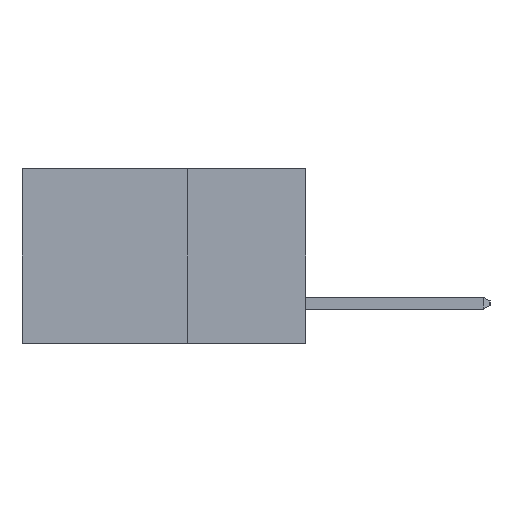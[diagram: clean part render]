
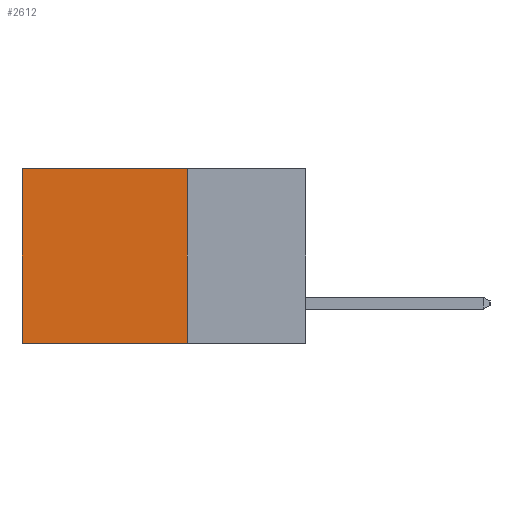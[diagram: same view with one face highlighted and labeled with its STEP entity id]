
A CAD part, left-side view. The second image highlights one B-rep face of the part: STEP entity #2612.
In plain terms, the highlighted planar face has unit normal (-1, 0, 0).
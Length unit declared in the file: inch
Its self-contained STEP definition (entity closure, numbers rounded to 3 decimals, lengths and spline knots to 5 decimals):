
#18 = CARTESIAN_POINT ( 'NONE',  ( 0.298, 0.25, 0. ) ) ;
#337 = DIRECTION ( 'NONE',  ( 0., 0., -1. ) ) ;
#370 = ORIENTED_EDGE ( 'NONE', *, *, #6235, .F. ) ;
#960 = DIRECTION ( 'NONE',  ( 0., 0., -1. ) ) ;
#2028 = VECTOR ( 'NONE', #3389, 39.37008 ) ;
#2294 = LINE ( 'NONE', #2478, #2028 ) ;
#2448 = FACE_OUTER_BOUND ( 'NONE', #9030, .T. ) ;
#2453 = PLANE ( 'NONE',  #4534 ) ;
#2478 = CARTESIAN_POINT ( 'NONE',  ( 0.298, 0.25, 0. ) ) ;
#2523 = CARTESIAN_POINT ( 'NONE',  ( 0.298, 0.6, -0.37 ) ) ;
#2564 = LINE ( 'NONE', #5707, #9399 ) ;
#2612 = ADVANCED_FACE ( 'NONE', ( #2448 ), #2453, .F. ) ;
#2887 = ORIENTED_EDGE ( 'NONE', *, *, #3330, .T. ) ;
#3072 = ORIENTED_EDGE ( 'NONE', *, *, #4757, .F. ) ;
#3108 = VERTEX_POINT ( 'NONE', #6675 ) ;
#3330 = EDGE_CURVE ( 'NONE', #3108, #5132, #2294, .T. ) ;
#3364 = DIRECTION ( 'NONE',  ( 1., 0., 0. ) ) ;
#3389 = DIRECTION ( 'NONE',  ( 0., 1., 0. ) ) ;
#3713 = EDGE_CURVE ( 'NONE', #5132, #5190, #2564, .T. ) ;
#4534 = AXIS2_PLACEMENT_3D ( 'NONE', #8694, #3364, #9599 ) ;
#4757 = EDGE_CURVE ( 'NONE', #3108, #4809, #10466, .T. ) ;
#4809 = VERTEX_POINT ( 'NONE', #7285 ) ;
#5132 = VERTEX_POINT ( 'NONE', #11326 ) ;
#5190 = VERTEX_POINT ( 'NONE', #2523 ) ;
#5590 = ORIENTED_EDGE ( 'NONE', *, *, #3713, .T. ) ;
#5707 = CARTESIAN_POINT ( 'NONE',  ( 0.298, 0.6, 0. ) ) ;
#5797 = DIRECTION ( 'NONE',  ( 0., 1., 0. ) ) ;
#6235 = EDGE_CURVE ( 'NONE', #4809, #5190, #8430, .T. ) ;
#6675 = CARTESIAN_POINT ( 'NONE',  ( 0.298, 0.25, 0. ) ) ;
#7285 = CARTESIAN_POINT ( 'NONE',  ( 0.298, 0.25, -0.37 ) ) ;
#8413 = VECTOR ( 'NONE', #960, 39.37008 ) ;
#8430 = LINE ( 'NONE', #9392, #10489 ) ;
#8694 = CARTESIAN_POINT ( 'NONE',  ( 0.298, 0.25, 0. ) ) ;
#9030 = EDGE_LOOP ( 'NONE', ( #5590, #370, #3072, #2887 ) ) ;
#9392 = CARTESIAN_POINT ( 'NONE',  ( 0.298, 0.25, -0.37 ) ) ;
#9399 = VECTOR ( 'NONE', #337, 39.37008 ) ;
#9599 = DIRECTION ( 'NONE',  ( 0., 0., -1. ) ) ;
#10466 = LINE ( 'NONE', #18, #8413 ) ;
#10489 = VECTOR ( 'NONE', #5797, 39.37008 ) ;
#11326 = CARTESIAN_POINT ( 'NONE',  ( 0.298, 0.6, 0. ) ) ;
